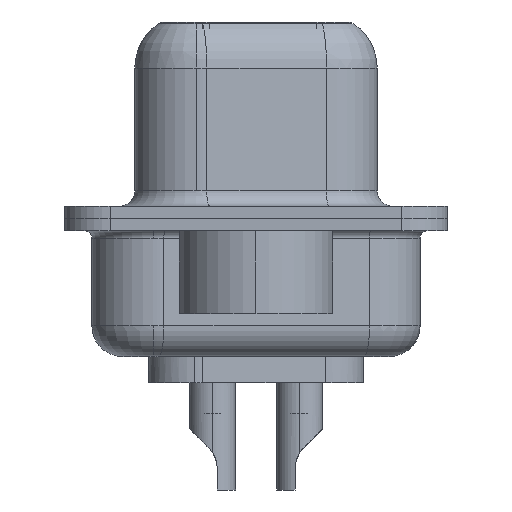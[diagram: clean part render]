
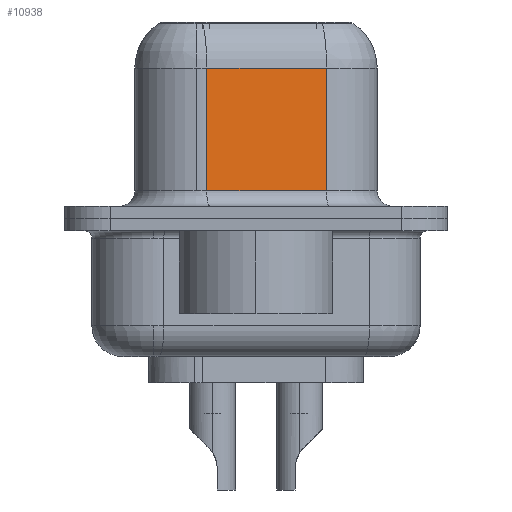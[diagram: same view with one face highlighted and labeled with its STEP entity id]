
A CAD part, left-side view. The second image highlights one B-rep face of the part: STEP entity #10938.
In plain terms, the highlighted planar face has unit normal (-0.985, -0.174, 0).
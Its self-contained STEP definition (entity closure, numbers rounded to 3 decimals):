
#282 = CARTESIAN_POINT ( 'NONE',  ( 5.068, -2.297, 6.65 ) ) ;
#1213 = LINE ( 'NONE', #19368, #8276 ) ;
#1443 = LINE ( 'NONE', #3081, #10362 ) ;
#2918 = LINE ( 'NONE', #11200, #15691 ) ;
#3081 = CARTESIAN_POINT ( 'NONE',  ( 4.38, 1.603, 6.65 ) ) ;
#3409 = CARTESIAN_POINT ( 'NONE',  ( 5.068, -2.297, 6.65 ) ) ;
#5026 = EDGE_CURVE ( 'NONE', #13956, #6747, #11550, .T. ) ;
#6747 = VERTEX_POINT ( 'NONE', #16790 ) ;
#6947 = ORIENTED_EDGE ( 'NONE', *, *, #23511, .T. ) ;
#7598 = CARTESIAN_POINT ( 'NONE',  ( 5.068, -2.297, 4.9 ) ) ;
#8276 = VECTOR ( 'NONE', #21404, 1000. ) ;
#8561 = DIRECTION ( 'NONE',  ( 0.985, 0.174, 0. ) ) ;
#8721 = EDGE_LOOP ( 'NONE', ( #17713, #18520, #16636, #6947 ) ) ;
#9629 = EDGE_CURVE ( 'NONE', #12562, #16503, #1443, .T. ) ;
#10362 = VECTOR ( 'NONE', #17839, 1000. ) ;
#10938 = ADVANCED_FACE ( 'NONE', ( #24915 ), #22906, .F. ) ;
#11200 = CARTESIAN_POINT ( 'NONE',  ( 5.068, -2.297, 0.9 ) ) ;
#11550 = LINE ( 'NONE', #3409, #22288 ) ;
#12251 = EDGE_CURVE ( 'NONE', #13956, #12562, #1213, .T. ) ;
#12562 = VERTEX_POINT ( 'NONE', #16521 ) ;
#13956 = VERTEX_POINT ( 'NONE', #7598 ) ;
#14308 = AXIS2_PLACEMENT_3D ( 'NONE', #282, #8561, #25050 ) ;
#15691 = VECTOR ( 'NONE', #22276, 1000. ) ;
#16503 = VERTEX_POINT ( 'NONE', #18235 ) ;
#16521 = CARTESIAN_POINT ( 'NONE',  ( 4.38, 1.603, 4.9 ) ) ;
#16636 = ORIENTED_EDGE ( 'NONE', *, *, #9629, .T. ) ;
#16790 = CARTESIAN_POINT ( 'NONE',  ( 5.068, -2.297, 0.9 ) ) ;
#17713 = ORIENTED_EDGE ( 'NONE', *, *, #5026, .F. ) ;
#17839 = DIRECTION ( 'NONE',  ( 0., 0., -1. ) ) ;
#18235 = CARTESIAN_POINT ( 'NONE',  ( 4.38, 1.603, 0.9 ) ) ;
#18520 = ORIENTED_EDGE ( 'NONE', *, *, #12251, .T. ) ;
#19368 = CARTESIAN_POINT ( 'NONE',  ( 5.068, -2.297, 4.9 ) ) ;
#21404 = DIRECTION ( 'NONE',  ( -0.174, 0.985, 0. ) ) ;
#22276 = DIRECTION ( 'NONE',  ( 0.174, -0.985, 0. ) ) ;
#22288 = VECTOR ( 'NONE', #24105, 1000. ) ;
#22906 = PLANE ( 'NONE',  #14308 ) ;
#23511 = EDGE_CURVE ( 'NONE', #16503, #6747, #2918, .T. ) ;
#24105 = DIRECTION ( 'NONE',  ( 0., 0., -1. ) ) ;
#24915 = FACE_OUTER_BOUND ( 'NONE', #8721, .T. ) ;
#25050 = DIRECTION ( 'NONE',  ( -0.174, 0.985, 0. ) ) ;
